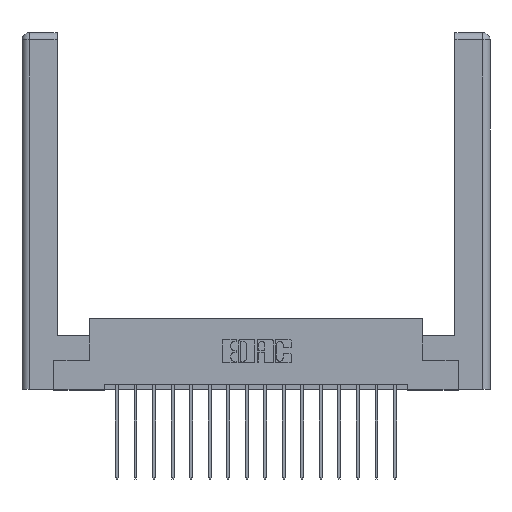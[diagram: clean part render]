
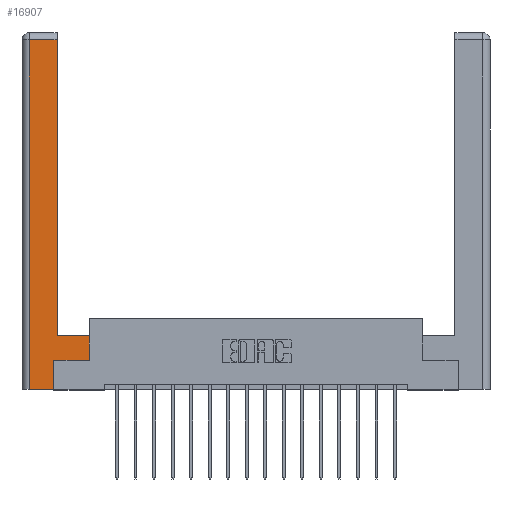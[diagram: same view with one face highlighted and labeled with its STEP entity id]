
A CAD part, top view. The second image highlights one B-rep face of the part: STEP entity #16907.
In plain terms, the highlighted planar face has unit normal (0, 0, 1).
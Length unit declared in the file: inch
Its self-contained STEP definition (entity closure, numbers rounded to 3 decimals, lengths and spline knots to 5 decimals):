
#344 = VECTOR ( 'NONE', #17939, 39.37008 ) ;
#357 = CARTESIAN_POINT ( 'NONE',  ( 0.565, 0.245, 0. ) ) ;
#648 = ORIENTED_EDGE ( 'NONE', *, *, #1410, .T. ) ;
#1245 = CARTESIAN_POINT ( 'NONE',  ( 0.265, 0., 0. ) ) ;
#1410 = EDGE_CURVE ( 'NONE', #7882, #16234, #18136, .T. ) ;
#2129 = LINE ( 'NONE', #6779, #16600 ) ;
#2193 = EDGE_CURVE ( 'NONE', #13168, #11776, #5416, .T. ) ;
#2388 = VERTEX_POINT ( 'NONE', #357 ) ;
#2696 = ORIENTED_EDGE ( 'NONE', *, *, #2193, .T. ) ;
#3000 = DIRECTION ( 'NONE',  ( -1., 0., 0. ) ) ;
#3902 = VECTOR ( 'NONE', #4076, 39.37008 ) ;
#3947 = EDGE_CURVE ( 'NONE', #16234, #2388, #7246, .T. ) ;
#4076 = DIRECTION ( 'NONE',  ( 1., 0., 0. ) ) ;
#4404 = ORIENTED_EDGE ( 'NONE', *, *, #13472, .T. ) ;
#4659 = PLANE ( 'NONE',  #6361 ) ;
#5233 = EDGE_CURVE ( 'NONE', #7990, #14828, #9363, .T. ) ;
#5416 = LINE ( 'NONE', #10624, #5884 ) ;
#5583 = CARTESIAN_POINT ( 'NONE',  ( 0.0615, 0., 0. ) ) ;
#5585 = VECTOR ( 'NONE', #3000, 39.37008 ) ;
#5653 = DIRECTION ( 'NONE',  ( 0., -1., 0. ) ) ;
#5884 = VECTOR ( 'NONE', #10743, 39.37008 ) ;
#6056 = DIRECTION ( 'NONE',  ( -1., 0., 0. ) ) ;
#6361 = AXIS2_PLACEMENT_3D ( 'NONE', #7282, #11734, #6056 ) ;
#6506 = ORIENTED_EDGE ( 'NONE', *, *, #9328, .T. ) ;
#6779 = CARTESIAN_POINT ( 'NONE',  ( 0.565, 0.45, 0. ) ) ;
#7120 = LINE ( 'NONE', #5583, #8671 ) ;
#7246 = LINE ( 'NONE', #15204, #344 ) ;
#7282 = CARTESIAN_POINT ( 'NONE',  ( 0., 0., 0. ) ) ;
#7664 = DIRECTION ( 'NONE',  ( 0., 1., 0. ) ) ;
#7734 = LINE ( 'NONE', #1245, #3902 ) ;
#7882 = VERTEX_POINT ( 'NONE', #9582 ) ;
#7990 = VERTEX_POINT ( 'NONE', #15950 ) ;
#8671 = VECTOR ( 'NONE', #5653, 39.37008 ) ;
#9038 = VECTOR ( 'NONE', #9907, 39.37008 ) ;
#9328 = EDGE_CURVE ( 'NONE', #2388, #13168, #2129, .T. ) ;
#9363 = LINE ( 'NONE', #11544, #5585 ) ;
#9582 = CARTESIAN_POINT ( 'NONE',  ( 0.265, 0., 0. ) ) ;
#9907 = DIRECTION ( 'NONE',  ( 0., 1., 0. ) ) ;
#10091 = ORIENTED_EDGE ( 'NONE', *, *, #3947, .T. ) ;
#10235 = ORIENTED_EDGE ( 'NONE', *, *, #5233, .T. ) ;
#10624 = CARTESIAN_POINT ( 'NONE',  ( 0.295, 0.45, 0. ) ) ;
#10743 = DIRECTION ( 'NONE',  ( -1., 0., 0. ) ) ;
#10916 = LINE ( 'NONE', #12820, #12930 ) ;
#10963 = VERTEX_POINT ( 'NONE', #15899 ) ;
#11083 = CARTESIAN_POINT ( 'NONE',  ( 0.265, 0.245, 0. ) ) ;
#11544 = CARTESIAN_POINT ( 'NONE',  ( 0.0615, 2.94, 0. ) ) ;
#11734 = DIRECTION ( 'NONE',  ( 0., 0., -1. ) ) ;
#11776 = VERTEX_POINT ( 'NONE', #16038 ) ;
#12351 = FACE_OUTER_BOUND ( 'NONE', #14037, .T. ) ;
#12820 = CARTESIAN_POINT ( 'NONE',  ( 0.295, 3., 0. ) ) ;
#12930 = VECTOR ( 'NONE', #7664, 39.37008 ) ;
#13162 = ORIENTED_EDGE ( 'NONE', *, *, #13830, .T. ) ;
#13168 = VERTEX_POINT ( 'NONE', #13844 ) ;
#13419 = CARTESIAN_POINT ( 'NONE',  ( 0.265, 0.245, 0. ) ) ;
#13472 = EDGE_CURVE ( 'NONE', #11776, #7990, #10916, .T. ) ;
#13830 = EDGE_CURVE ( 'NONE', #14828, #10963, #7120, .T. ) ;
#13844 = CARTESIAN_POINT ( 'NONE',  ( 0.565, 0.45, 0. ) ) ;
#14037 = EDGE_LOOP ( 'NONE', ( #4404, #10235, #13162, #15247, #648, #10091, #6506, #2696 ) ) ;
#14828 = VERTEX_POINT ( 'NONE', #16537 ) ;
#15204 = CARTESIAN_POINT ( 'NONE',  ( 0.565, 0.245, 0. ) ) ;
#15247 = ORIENTED_EDGE ( 'NONE', *, *, #15275, .T. ) ;
#15275 = EDGE_CURVE ( 'NONE', #10963, #7882, #7734, .T. ) ;
#15899 = CARTESIAN_POINT ( 'NONE',  ( 0.0615, 0., 0. ) ) ;
#15950 = CARTESIAN_POINT ( 'NONE',  ( 0.295, 2.94, 0. ) ) ;
#16038 = CARTESIAN_POINT ( 'NONE',  ( 0.295, 0.45, 0. ) ) ;
#16234 = VERTEX_POINT ( 'NONE', #13419 ) ;
#16537 = CARTESIAN_POINT ( 'NONE',  ( 0.0615, 2.94, 0. ) ) ;
#16600 = VECTOR ( 'NONE', #16659, 39.37008 ) ;
#16659 = DIRECTION ( 'NONE',  ( 0., 1., 0. ) ) ;
#16907 = ADVANCED_FACE ( 'NONE', ( #12351 ), #4659, .F. ) ;
#17939 = DIRECTION ( 'NONE',  ( 1., 0., 0. ) ) ;
#18136 = LINE ( 'NONE', #11083, #9038 ) ;
